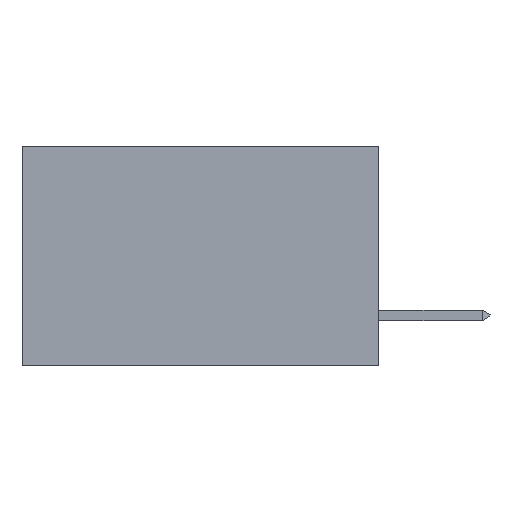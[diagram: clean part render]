
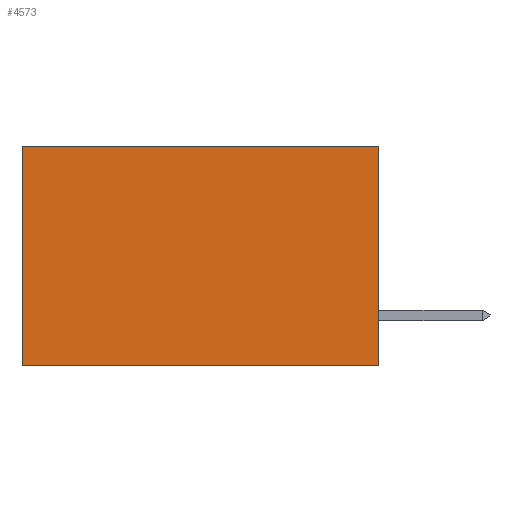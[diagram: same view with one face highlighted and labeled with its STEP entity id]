
A CAD part, left-side view. The second image highlights one B-rep face of the part: STEP entity #4573.
In plain terms, the highlighted planar face has unit normal (-1, 0, 0).
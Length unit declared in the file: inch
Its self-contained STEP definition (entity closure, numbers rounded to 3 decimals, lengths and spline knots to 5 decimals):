
#1283 = CARTESIAN_POINT ( 'NONE',  ( 0.298, 0.6, 0. ) ) ;
#2375 = FACE_OUTER_BOUND ( 'NONE', #14391, .T. ) ;
#2992 = VECTOR ( 'NONE', #6013, 39.37008 ) ;
#3117 = EDGE_CURVE ( 'NONE', #6301, #15166, #12493, .T. ) ;
#3227 = DIRECTION ( 'NONE',  ( 0., 0., -1. ) ) ;
#3591 = CARTESIAN_POINT ( 'NONE',  ( 0.298, 0.6, 0. ) ) ;
#4147 = ORIENTED_EDGE ( 'NONE', *, *, #6874, .F. ) ;
#4573 = ADVANCED_FACE ( 'NONE', ( #2375 ), #12968, .F. ) ;
#5754 = LINE ( 'NONE', #15686, #8635 ) ;
#6013 = DIRECTION ( 'NONE',  ( 0., 0., -1. ) ) ;
#6301 = VERTEX_POINT ( 'NONE', #1283 ) ;
#6615 = AXIS2_PLACEMENT_3D ( 'NONE', #6841, #11813, #3227 ) ;
#6841 = CARTESIAN_POINT ( 'NONE',  ( 0.298, 0., 0. ) ) ;
#6874 = EDGE_CURVE ( 'NONE', #11534, #15166, #11665, .T. ) ;
#7121 = DIRECTION ( 'NONE',  ( 0., 1., 0. ) ) ;
#8227 = VERTEX_POINT ( 'NONE', #9922 ) ;
#8459 = CARTESIAN_POINT ( 'NONE',  ( 0.298, 0., 0. ) ) ;
#8635 = VECTOR ( 'NONE', #7121, 39.37008 ) ;
#9166 = EDGE_CURVE ( 'NONE', #8227, #6301, #5754, .T. ) ;
#9922 = CARTESIAN_POINT ( 'NONE',  ( 0.298, 0., 0. ) ) ;
#10105 = LINE ( 'NONE', #8459, #13852 ) ;
#10279 = CARTESIAN_POINT ( 'NONE',  ( 0.298, 0.6, -0.37 ) ) ;
#10451 = CARTESIAN_POINT ( 'NONE',  ( 0.298, 0., -0.37 ) ) ;
#10934 = CARTESIAN_POINT ( 'NONE',  ( 0.298, 0., -0.37 ) ) ;
#11441 = EDGE_CURVE ( 'NONE', #8227, #11534, #10105, .T. ) ;
#11470 = VECTOR ( 'NONE', #13311, 39.37008 ) ;
#11528 = DIRECTION ( 'NONE',  ( 0., 0., -1. ) ) ;
#11534 = VERTEX_POINT ( 'NONE', #10451 ) ;
#11665 = LINE ( 'NONE', #10934, #11470 ) ;
#11813 = DIRECTION ( 'NONE',  ( 1., 0., 0. ) ) ;
#12283 = ORIENTED_EDGE ( 'NONE', *, *, #3117, .T. ) ;
#12493 = LINE ( 'NONE', #3591, #2992 ) ;
#12968 = PLANE ( 'NONE',  #6615 ) ;
#13311 = DIRECTION ( 'NONE',  ( 0., 1., 0. ) ) ;
#13506 = ORIENTED_EDGE ( 'NONE', *, *, #9166, .T. ) ;
#13852 = VECTOR ( 'NONE', #11528, 39.37008 ) ;
#14109 = ORIENTED_EDGE ( 'NONE', *, *, #11441, .F. ) ;
#14391 = EDGE_LOOP ( 'NONE', ( #12283, #4147, #14109, #13506 ) ) ;
#15166 = VERTEX_POINT ( 'NONE', #10279 ) ;
#15686 = CARTESIAN_POINT ( 'NONE',  ( 0.298, 0., 0. ) ) ;
